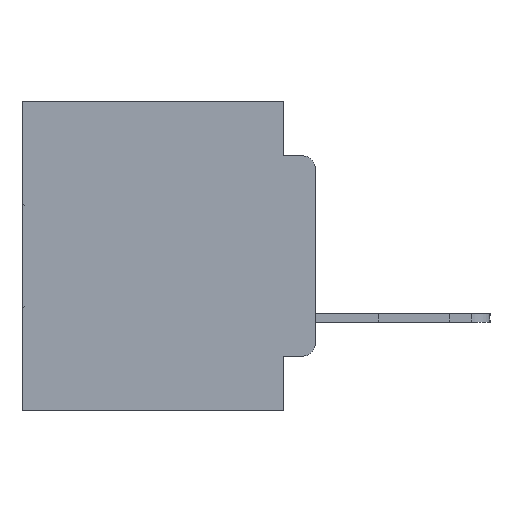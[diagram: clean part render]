
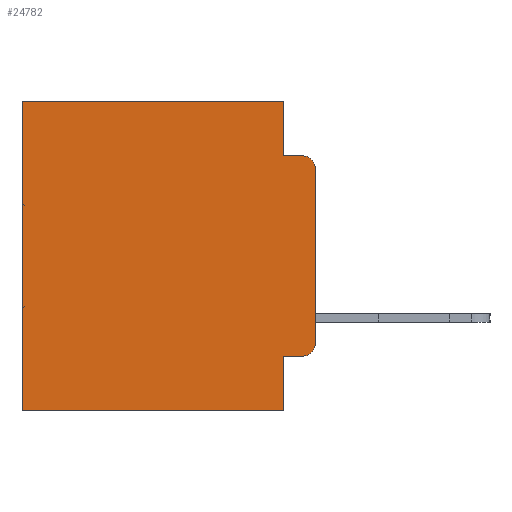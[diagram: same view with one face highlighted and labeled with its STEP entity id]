
A CAD part, left-side view. The second image highlights one B-rep face of the part: STEP entity #24782.
In plain terms, the highlighted planar face has unit normal (-1, 0, 0).
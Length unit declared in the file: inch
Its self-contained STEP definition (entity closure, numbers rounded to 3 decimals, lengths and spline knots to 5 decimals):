
#536 = LINE ( 'NONE', #12474, #19439 ) ;
#729 = CARTESIAN_POINT ( 'NONE',  ( 0.298, 0., 0. ) ) ;
#1537 = EDGE_CURVE ( 'NONE', #12868, #31109, #4438, .T. ) ;
#2671 = VERTEX_POINT ( 'NONE', #30161 ) ;
#3086 = EDGE_CURVE ( 'NONE', #16989, #31802, #23519, .T. ) ;
#3100 = CARTESIAN_POINT ( 'NONE',  ( 0.298, 0.051, -0.4115 ) ) ;
#3259 = DIRECTION ( 'NONE',  ( 0., 0., -1. ) ) ;
#3518 = EDGE_CURVE ( 'NONE', #19075, #19562, #12079, .T. ) ;
#3649 = VECTOR ( 'NONE', #21387, 39.37008 ) ;
#3751 = AXIS2_PLACEMENT_3D ( 'NONE', #729, #18013, #3259 ) ;
#3917 = LINE ( 'NONE', #24149, #9057 ) ;
#4250 = DIRECTION ( 'NONE',  ( 0., 0., -1. ) ) ;
#4319 = EDGE_LOOP ( 'NONE', ( #6701, #13216, #9806, #24257, #12075, #12848, #16647, #25718, #5912, #18928 ) ) ;
#4438 = LINE ( 'NONE', #14926, #3649 ) ;
#4695 = VECTOR ( 'NONE', #4250, 39.37008 ) ;
#4763 = EDGE_CURVE ( 'NONE', #27957, #31802, #24928, .T. ) ;
#5912 = ORIENTED_EDGE ( 'NONE', *, *, #16134, .T. ) ;
#6037 = VECTOR ( 'NONE', #23479, 39.37008 ) ;
#6269 = CARTESIAN_POINT ( 'NONE',  ( 0.298, 0.02, -0.3915 ) ) ;
#6701 = ORIENTED_EDGE ( 'NONE', *, *, #26210, .F. ) ;
#6782 = CARTESIAN_POINT ( 'NONE',  ( 0.298, 0.02, -0.0885 ) ) ;
#8172 = LINE ( 'NONE', #19194, #26722 ) ;
#8419 = AXIS2_PLACEMENT_3D ( 'NONE', #6269, #23347, #8803 ) ;
#8803 = DIRECTION ( 'NONE',  ( 0., 0., -1. ) ) ;
#9057 = VECTOR ( 'NONE', #9600, 39.37008 ) ;
#9391 = CARTESIAN_POINT ( 'NONE',  ( 0.298, 0.051, 0. ) ) ;
#9600 = DIRECTION ( 'NONE',  ( 0., 1., 0. ) ) ;
#9806 = ORIENTED_EDGE ( 'NONE', *, *, #4763, .F. ) ;
#11455 = VECTOR ( 'NONE', #27561, 39.37008 ) ;
#11772 = DIRECTION ( 'NONE',  ( -1., 0., 0. ) ) ;
#11818 = DIRECTION ( 'NONE',  ( 0., 0., -1. ) ) ;
#12075 = ORIENTED_EDGE ( 'NONE', *, *, #1537, .T. ) ;
#12079 = LINE ( 'NONE', #28809, #4695 ) ;
#12386 = VERTEX_POINT ( 'NONE', #13680 ) ;
#12474 = CARTESIAN_POINT ( 'NONE',  ( 0.298, 0.473, 0. ) ) ;
#12848 = ORIENTED_EDGE ( 'NONE', *, *, #28697, .T. ) ;
#12868 = VERTEX_POINT ( 'NONE', #9391 ) ;
#13216 = ORIENTED_EDGE ( 'NONE', *, *, #3086, .T. ) ;
#13680 = CARTESIAN_POINT ( 'NONE',  ( 0.298, 0., -0.3915 ) ) ;
#14228 = CARTESIAN_POINT ( 'NONE',  ( 0.298, 0.051, -0.0885 ) ) ;
#14926 = CARTESIAN_POINT ( 'NONE',  ( 0.298, 0., 0. ) ) ;
#14929 = DIRECTION ( 'NONE',  ( 0., 0., -1. ) ) ;
#15160 = CIRCLE ( 'NONE', #8419, 0.02 ) ;
#16134 = EDGE_CURVE ( 'NONE', #19075, #26836, #17926, .T. ) ;
#16310 = EDGE_CURVE ( 'NONE', #12868, #27957, #19803, .T. ) ;
#16647 = ORIENTED_EDGE ( 'NONE', *, *, #23001, .F. ) ;
#16876 = CARTESIAN_POINT ( 'NONE',  ( 0.298, 0.051, -0.0885 ) ) ;
#16989 = VERTEX_POINT ( 'NONE', #26036 ) ;
#17926 = LINE ( 'NONE', #3100, #11455 ) ;
#18013 = DIRECTION ( 'NONE',  ( 1., 0., 0. ) ) ;
#18928 = ORIENTED_EDGE ( 'NONE', *, *, #24299, .T. ) ;
#19075 = VERTEX_POINT ( 'NONE', #21459 ) ;
#19194 = CARTESIAN_POINT ( 'NONE',  ( 0.298, 0., 0. ) ) ;
#19439 = VECTOR ( 'NONE', #14929, 39.37008 ) ;
#19562 = VERTEX_POINT ( 'NONE', #31223 ) ;
#19803 = LINE ( 'NONE', #20998, #6037 ) ;
#20336 = PLANE ( 'NONE',  #3751 ) ;
#20609 = AXIS2_PLACEMENT_3D ( 'NONE', #22685, #11772, #11818 ) ;
#20998 = CARTESIAN_POINT ( 'NONE',  ( 0.298, 0.051, 0. ) ) ;
#21387 = DIRECTION ( 'NONE',  ( 0., 1., 0. ) ) ;
#21459 = CARTESIAN_POINT ( 'NONE',  ( 0.298, 0.051, -0.4115 ) ) ;
#21613 = DIRECTION ( 'NONE',  ( 0., 0., -1. ) ) ;
#22685 = CARTESIAN_POINT ( 'NONE',  ( 0.298, 0.02, -0.1085 ) ) ;
#23001 = EDGE_CURVE ( 'NONE', #19562, #2671, #3917, .T. ) ;
#23347 = DIRECTION ( 'NONE',  ( -1., 0., 0. ) ) ;
#23479 = DIRECTION ( 'NONE',  ( 0., 0., -1. ) ) ;
#23519 = CIRCLE ( 'NONE', #20609, 0.02 ) ;
#24149 = CARTESIAN_POINT ( 'NONE',  ( 0.298, 0., -0.5 ) ) ;
#24257 = ORIENTED_EDGE ( 'NONE', *, *, #16310, .F. ) ;
#24299 = EDGE_CURVE ( 'NONE', #26836, #12386, #15160, .T. ) ;
#24782 = ADVANCED_FACE ( 'NONE', ( #24990 ), #20336, .F. ) ;
#24928 = LINE ( 'NONE', #14228, #25637 ) ;
#24990 = FACE_OUTER_BOUND ( 'NONE', #4319, .T. ) ;
#25637 = VECTOR ( 'NONE', #28724, 39.37008 ) ;
#25718 = ORIENTED_EDGE ( 'NONE', *, *, #3518, .F. ) ;
#26036 = CARTESIAN_POINT ( 'NONE',  ( 0.298, 0., -0.1085 ) ) ;
#26210 = EDGE_CURVE ( 'NONE', #16989, #12386, #8172, .T. ) ;
#26722 = VECTOR ( 'NONE', #21613, 39.37008 ) ;
#26836 = VERTEX_POINT ( 'NONE', #31597 ) ;
#27561 = DIRECTION ( 'NONE',  ( 0., -1., 0. ) ) ;
#27957 = VERTEX_POINT ( 'NONE', #16876 ) ;
#28697 = EDGE_CURVE ( 'NONE', #31109, #2671, #536, .T. ) ;
#28724 = DIRECTION ( 'NONE',  ( 0., -1., 0. ) ) ;
#28809 = CARTESIAN_POINT ( 'NONE',  ( 0.298, 0.051, 0. ) ) ;
#30161 = CARTESIAN_POINT ( 'NONE',  ( 0.298, 0.473, -0.5 ) ) ;
#30947 = CARTESIAN_POINT ( 'NONE',  ( 0.298, 0.473, 0. ) ) ;
#31109 = VERTEX_POINT ( 'NONE', #30947 ) ;
#31223 = CARTESIAN_POINT ( 'NONE',  ( 0.298, 0.051, -0.5 ) ) ;
#31597 = CARTESIAN_POINT ( 'NONE',  ( 0.298, 0.02, -0.4115 ) ) ;
#31802 = VERTEX_POINT ( 'NONE', #6782 ) ;
